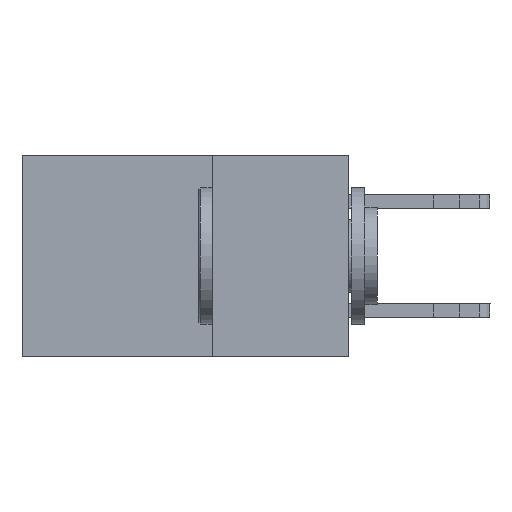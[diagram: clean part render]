
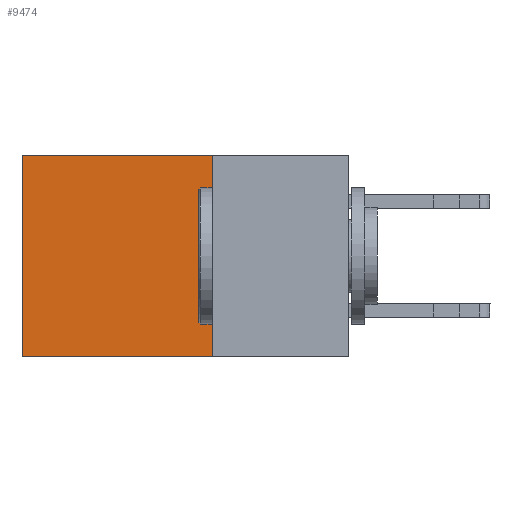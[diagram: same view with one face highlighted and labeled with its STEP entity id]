
A CAD part, left-side view. The second image highlights one B-rep face of the part: STEP entity #9474.
In plain terms, the highlighted planar face has unit normal (-1, 0, 0).
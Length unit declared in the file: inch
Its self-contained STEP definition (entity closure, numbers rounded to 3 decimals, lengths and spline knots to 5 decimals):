
#790 = VECTOR ( 'NONE', #4648, 39.37008 ) ;
#831 = LINE ( 'NONE', #18073, #19530 ) ;
#1718 = DIRECTION ( 'NONE',  ( 0., 0., -1. ) ) ;
#2437 = PLANE ( 'NONE',  #10107 ) ;
#3765 = EDGE_CURVE ( 'NONE', #8968, #11214, #16660, .T. ) ;
#3886 = DIRECTION ( 'NONE',  ( 0., 0., -1. ) ) ;
#4013 = CARTESIAN_POINT ( 'NONE',  ( 0.298, 0.6, -0.37 ) ) ;
#4111 = ORIENTED_EDGE ( 'NONE', *, *, #3765, .T. ) ;
#4648 = DIRECTION ( 'NONE',  ( 0., 1., 0. ) ) ;
#4701 = LINE ( 'NONE', #18252, #16294 ) ;
#5965 = CARTESIAN_POINT ( 'NONE',  ( 0.298, 0.6, 0. ) ) ;
#6052 = CARTESIAN_POINT ( 'NONE',  ( 0.298, 0.25, 0. ) ) ;
#6864 = CARTESIAN_POINT ( 'NONE',  ( 0.298, 0.25, 0. ) ) ;
#7058 = DIRECTION ( 'NONE',  ( 1., 0., 0. ) ) ;
#7143 = ORIENTED_EDGE ( 'NONE', *, *, #15280, .F. ) ;
#7777 = CARTESIAN_POINT ( 'NONE',  ( 0.298, 0.25, 0. ) ) ;
#8643 = FACE_OUTER_BOUND ( 'NONE', #15069, .T. ) ;
#8968 = VERTEX_POINT ( 'NONE', #6052 ) ;
#9059 = ORIENTED_EDGE ( 'NONE', *, *, #19160, .F. ) ;
#9474 = ADVANCED_FACE ( 'NONE', ( #8643 ), #2437, .F. ) ;
#10107 = AXIS2_PLACEMENT_3D ( 'NONE', #15968, #7058, #15901 ) ;
#10787 = VERTEX_POINT ( 'NONE', #4013 ) ;
#11214 = VERTEX_POINT ( 'NONE', #5965 ) ;
#11548 = VECTOR ( 'NONE', #3886, 39.37008 ) ;
#12512 = LINE ( 'NONE', #6864, #11548 ) ;
#13736 = EDGE_CURVE ( 'NONE', #11214, #10787, #4701, .T. ) ;
#15069 = EDGE_LOOP ( 'NONE', ( #18465, #7143, #9059, #4111 ) ) ;
#15280 = EDGE_CURVE ( 'NONE', #16473, #10787, #831, .T. ) ;
#15901 = DIRECTION ( 'NONE',  ( 0., 0., -1. ) ) ;
#15968 = CARTESIAN_POINT ( 'NONE',  ( 0.298, 0.25, 0. ) ) ;
#16294 = VECTOR ( 'NONE', #1718, 39.37008 ) ;
#16473 = VERTEX_POINT ( 'NONE', #18631 ) ;
#16660 = LINE ( 'NONE', #7777, #790 ) ;
#18073 = CARTESIAN_POINT ( 'NONE',  ( 0.298, 0.25, -0.37 ) ) ;
#18252 = CARTESIAN_POINT ( 'NONE',  ( 0.298, 0.6, 0. ) ) ;
#18465 = ORIENTED_EDGE ( 'NONE', *, *, #13736, .T. ) ;
#18631 = CARTESIAN_POINT ( 'NONE',  ( 0.298, 0.25, -0.37 ) ) ;
#18888 = DIRECTION ( 'NONE',  ( 0., 1., 0. ) ) ;
#19160 = EDGE_CURVE ( 'NONE', #8968, #16473, #12512, .T. ) ;
#19530 = VECTOR ( 'NONE', #18888, 39.37008 ) ;
